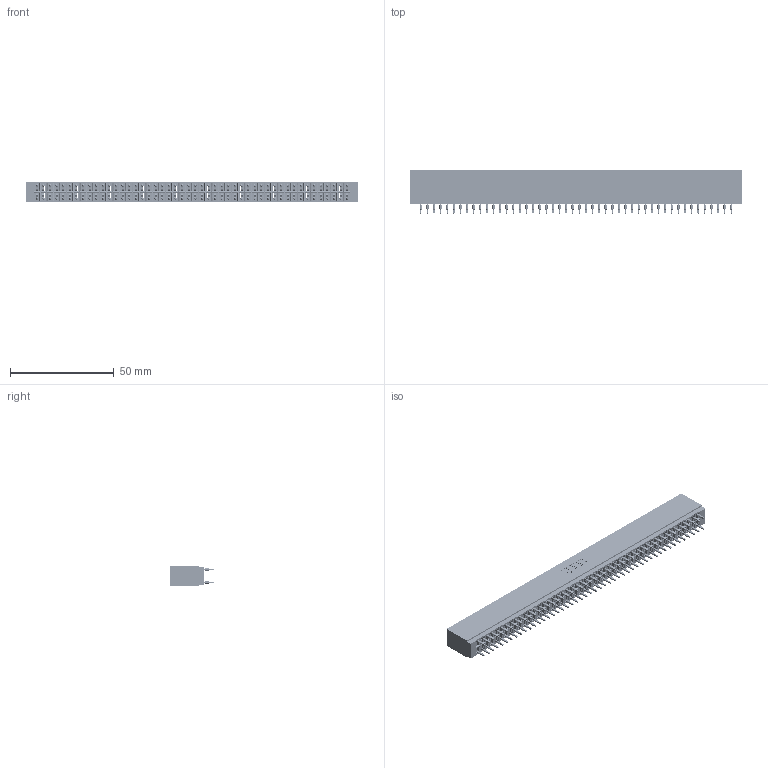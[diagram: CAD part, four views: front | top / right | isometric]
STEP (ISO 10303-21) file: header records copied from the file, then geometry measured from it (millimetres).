
FILE_DESCRIPTION (( 'STEP AP203' ), '1' );
FILE_NAME ('746-096-560-201.STEP', '2026-03-04T21:42:42', ( '' ), ( '' ), 'SwSTEP 2.0', 'SolidWorks 2023', '' );
FILE_SCHEMA (( 'CONFIG_CONTROL_DESIGN' ));
Length unit declared in the file: millimetre
Products named in the file (3): 746-292-001_560; 746-096-560-201; 746 Part_.515 Slot Depth - 01
Assembly tree (97 placements, depth 2):
  746-096-560-201
    746 Part_.515 Slot Depth - 01
    746-292-001_560  x96
Bounding box: 159.64 x 20.82 x 9.91 mm (x, y, z)
Volume: 17405.5 mm3; surface area: 29634.7 mm2
Topology: 97 solids, 97 shells, 9169 faces, 25511 edges, 16351 vertices
Faces by surface type: plane 4567, cylinder 2106, bspline 1920, torus 576
Entity records: 73412 total; most frequent: CARTESIAN_POINT 14539, ORIENTED_EDGE 12642, DIRECTION 10551, EDGE_CURVE 6321, LINE 5649, VECTOR 5649, VERTEX_POINT 4191, AXIS2_PLACEMENT_3D 2451
